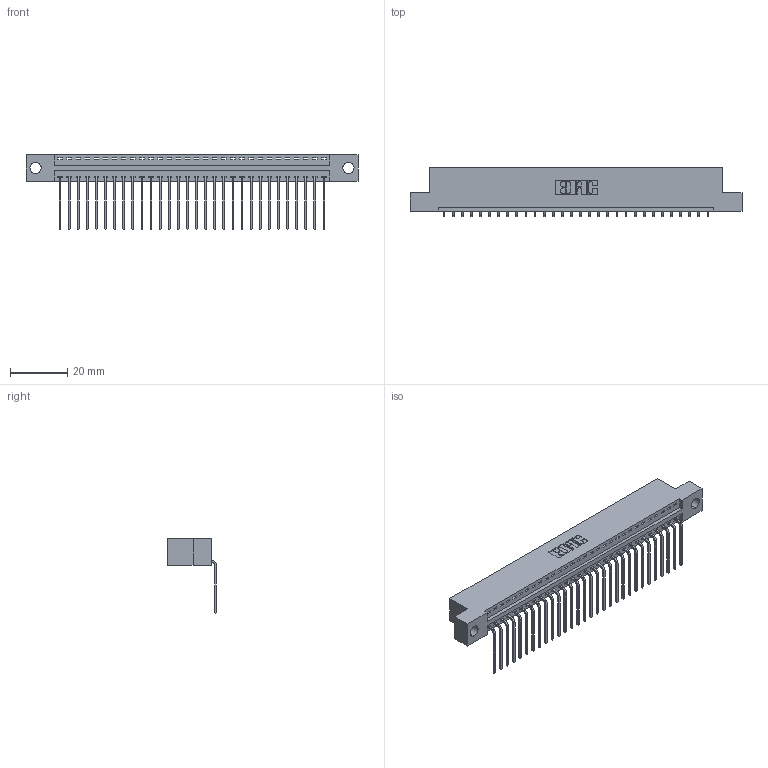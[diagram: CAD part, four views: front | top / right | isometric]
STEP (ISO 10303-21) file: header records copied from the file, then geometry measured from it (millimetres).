
FILE_DESCRIPTION (( 'STEP AP203' ), '1' );
FILE_NAME ('396-030-559-104.STEP', '2019-10-31T21:48:00', ( '' ), ( '' ), 'SwSTEP 2.0', 'SolidWorks 2016', '' );
FILE_SCHEMA (( 'CONFIG_CONTROL_DESIGN' ));
Length unit declared in the file: inch
Products named in the file (3): 345-292-001_558 559 Tail - 1; 396-030-559-104; 346 Part_Flush Mounting Lugs - 0.156 Dia-TH
Assembly tree (31 placements, depth 2):
  396-030-559-104
    346 Part_Flush Mounting Lugs - 0.156 Dia-TH
    345-292-001_558 559 Tail - 1  x30
Bounding box: 115.82 x 17.08 x 26.16 mm (x, y, z)
Volume: 11016.3 mm3; surface area: 14040.8 mm2
Topology: 31 solids, 31 shells, 1922 faces, 5789 edges, 3818 vertices
Faces by surface type: plane 1336, cylinder 586
Entity records: 20321 total; most frequent: CARTESIAN_POINT 3494, ORIENTED_EDGE 3458, DIRECTION 3097, EDGE_CURVE 1729, LINE 1477, VECTOR 1477, VERTEX_POINT 1150, AXIS2_PLACEMENT_3D 810
